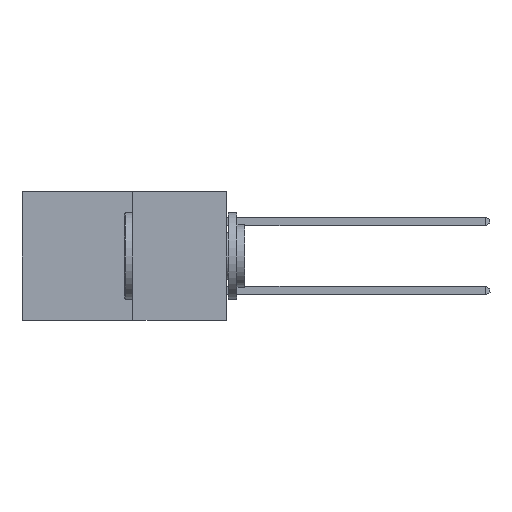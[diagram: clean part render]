
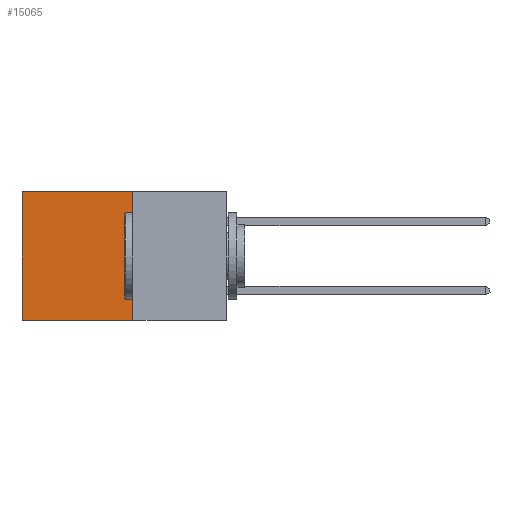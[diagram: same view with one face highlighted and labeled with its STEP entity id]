
A CAD part, left-side view. The second image highlights one B-rep face of the part: STEP entity #15065.
In plain terms, the highlighted planar face has unit normal (-1, 0, 0).
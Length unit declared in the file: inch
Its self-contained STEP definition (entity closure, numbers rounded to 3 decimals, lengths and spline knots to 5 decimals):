
#205 = CARTESIAN_POINT ( 'NONE',  ( 0.277, 0.27, 0. ) ) ;
#2312 = VECTOR ( 'NONE', #7038, 39.37008 ) ;
#2512 = EDGE_CURVE ( 'NONE', #23798, #14053, #22337, .T. ) ;
#2585 = DIRECTION ( 'NONE',  ( 0., 0., -1. ) ) ;
#3552 = VERTEX_POINT ( 'NONE', #16908 ) ;
#4177 = CARTESIAN_POINT ( 'NONE',  ( 0.277, 0.59, -0.37 ) ) ;
#4442 = CARTESIAN_POINT ( 'NONE',  ( 0.277, 0.27, -0.37 ) ) ;
#5723 = EDGE_CURVE ( 'NONE', #14053, #23314, #22941, .T. ) ;
#7038 = DIRECTION ( 'NONE',  ( 0., 1., 0. ) ) ;
#8365 = DIRECTION ( 'NONE',  ( 0., 1., 0. ) ) ;
#9617 = ORIENTED_EDGE ( 'NONE', *, *, #5723, .F. ) ;
#11807 = DIRECTION ( 'NONE',  ( 0., 0., -1. ) ) ;
#11912 = FACE_OUTER_BOUND ( 'NONE', #24239, .T. ) ;
#14053 = VERTEX_POINT ( 'NONE', #4442 ) ;
#15065 = ADVANCED_FACE ( 'NONE', ( #11912 ), #34536, .F. ) ;
#15197 = CARTESIAN_POINT ( 'NONE',  ( 0.277, 0.27, -0.37 ) ) ;
#16062 = CARTESIAN_POINT ( 'NONE',  ( 0.277, 0.27, -0.37 ) ) ;
#16663 = ORIENTED_EDGE ( 'NONE', *, *, #26480, .T. ) ;
#16908 = CARTESIAN_POINT ( 'NONE',  ( 0.277, 0.59, 0. ) ) ;
#17232 = LINE ( 'NONE', #205, #25098 ) ;
#18757 = DIRECTION ( 'NONE',  ( 1., 0., 0. ) ) ;
#21505 = VECTOR ( 'NONE', #31242, 39.37008 ) ;
#22337 = LINE ( 'NONE', #29576, #21505 ) ;
#22404 = CARTESIAN_POINT ( 'NONE',  ( 0.277, 0.27, 0. ) ) ;
#22941 = LINE ( 'NONE', #15197, #2312 ) ;
#23177 = ORIENTED_EDGE ( 'NONE', *, *, #2512, .F. ) ;
#23190 = ORIENTED_EDGE ( 'NONE', *, *, #24046, .T. ) ;
#23314 = VERTEX_POINT ( 'NONE', #4177 ) ;
#23798 = VERTEX_POINT ( 'NONE', #22404 ) ;
#24046 = EDGE_CURVE ( 'NONE', #3552, #23314, #34362, .T. ) ;
#24239 = EDGE_LOOP ( 'NONE', ( #23190, #9617, #23177, #16663 ) ) ;
#24347 = AXIS2_PLACEMENT_3D ( 'NONE', #16062, #18757, #2585 ) ;
#25098 = VECTOR ( 'NONE', #8365, 39.37008 ) ;
#26480 = EDGE_CURVE ( 'NONE', #23798, #3552, #17232, .T. ) ;
#28202 = VECTOR ( 'NONE', #11807, 39.37008 ) ;
#29576 = CARTESIAN_POINT ( 'NONE',  ( 0.277, 0.27, -0.37 ) ) ;
#30443 = CARTESIAN_POINT ( 'NONE',  ( 0.277, 0.59, -0.37 ) ) ;
#31242 = DIRECTION ( 'NONE',  ( 0., 0., -1. ) ) ;
#34362 = LINE ( 'NONE', #30443, #28202 ) ;
#34536 = PLANE ( 'NONE',  #24347 ) ;
